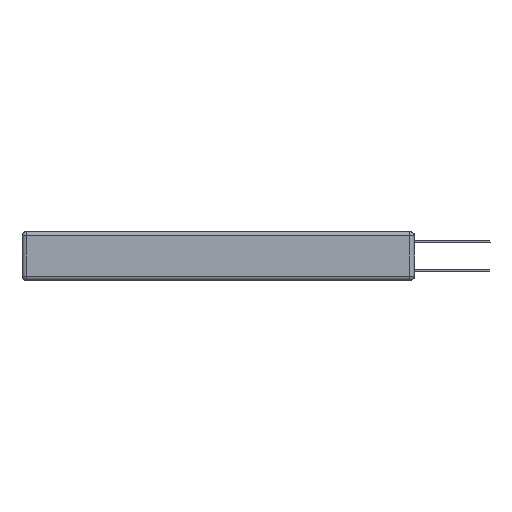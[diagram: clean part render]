
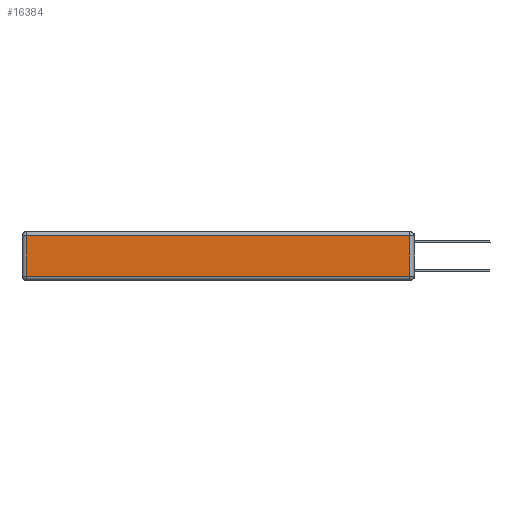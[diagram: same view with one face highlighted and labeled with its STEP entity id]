
A CAD part, left-side view. The second image highlights one B-rep face of the part: STEP entity #16384.
In plain terms, the highlighted planar face has unit normal (-1, 0, 0).
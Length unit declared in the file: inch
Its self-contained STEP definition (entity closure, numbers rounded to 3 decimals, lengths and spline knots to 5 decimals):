
#1165 = DIRECTION ( 'NONE',  ( 0., 0., -1. ) ) ;
#2131 = CARTESIAN_POINT ( 'NONE',  ( 0., 2.72, -0.03 ) ) ;
#2928 = ORIENTED_EDGE ( 'NONE', *, *, #4893, .T. ) ;
#3922 = EDGE_CURVE ( 'NONE', #14248, #5487, #15066, .T. ) ;
#4221 = EDGE_CURVE ( 'NONE', #5487, #18503, #12332, .T. ) ;
#4314 = CARTESIAN_POINT ( 'NONE',  ( 0., 2.72, -0.313 ) ) ;
#4434 = CARTESIAN_POINT ( 'NONE',  ( 0., 0., -0.343 ) ) ;
#4870 = VECTOR ( 'NONE', #14409, 39.37008 ) ;
#4893 = EDGE_CURVE ( 'NONE', #18503, #14040, #14017, .T. ) ;
#5487 = VERTEX_POINT ( 'NONE', #17688 ) ;
#6103 = ORIENTED_EDGE ( 'NONE', *, *, #3922, .T. ) ;
#6251 = DIRECTION ( 'NONE',  ( -1., 0., 0. ) ) ;
#6723 = ORIENTED_EDGE ( 'NONE', *, *, #9563, .T. ) ;
#8001 = EDGE_LOOP ( 'NONE', ( #6103, #8261, #2928, #6723 ) ) ;
#8261 = ORIENTED_EDGE ( 'NONE', *, *, #4221, .T. ) ;
#9563 = EDGE_CURVE ( 'NONE', #14040, #14248, #19820, .T. ) ;
#9757 = CARTESIAN_POINT ( 'NONE',  ( 0., 2.75, -0.03 ) ) ;
#10642 = PLANE ( 'NONE',  #11002 ) ;
#10918 = VECTOR ( 'NONE', #19430, 39.37008 ) ;
#11002 = AXIS2_PLACEMENT_3D ( 'NONE', #4434, #6251, #13751 ) ;
#11413 = CARTESIAN_POINT ( 'NONE',  ( 0., 0.03, -0.343 ) ) ;
#12198 = VECTOR ( 'NONE', #1165, 39.37008 ) ;
#12332 = LINE ( 'NONE', #11413, #4870 ) ;
#13024 = VECTOR ( 'NONE', #15854, 39.37008 ) ;
#13751 = DIRECTION ( 'NONE',  ( 0., 0., 1. ) ) ;
#14017 = LINE ( 'NONE', #9757, #13024 ) ;
#14040 = VERTEX_POINT ( 'NONE', #2131 ) ;
#14248 = VERTEX_POINT ( 'NONE', #4314 ) ;
#14409 = DIRECTION ( 'NONE',  ( 0., 0., 1. ) ) ;
#14835 = CARTESIAN_POINT ( 'NONE',  ( 0., 0., -0.313 ) ) ;
#15066 = LINE ( 'NONE', #14835, #10918 ) ;
#15854 = DIRECTION ( 'NONE',  ( 0., 1., 0. ) ) ;
#16384 = ADVANCED_FACE ( 'NONE', ( #17903 ), #10642, .T. ) ;
#17188 = CARTESIAN_POINT ( 'NONE',  ( 0., 0.03, -0.03 ) ) ;
#17688 = CARTESIAN_POINT ( 'NONE',  ( 0., 0.03, -0.313 ) ) ;
#17903 = FACE_OUTER_BOUND ( 'NONE', #8001, .T. ) ;
#18503 = VERTEX_POINT ( 'NONE', #17188 ) ;
#19430 = DIRECTION ( 'NONE',  ( 0., -1., 0. ) ) ;
#19753 = CARTESIAN_POINT ( 'NONE',  ( 0., 2.72, -0.343 ) ) ;
#19820 = LINE ( 'NONE', #19753, #12198 ) ;
